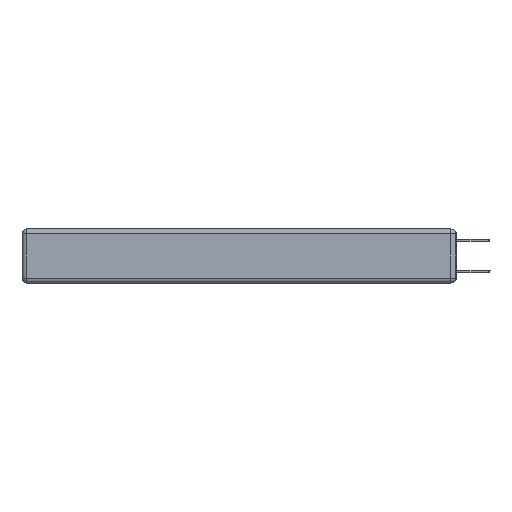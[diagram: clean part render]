
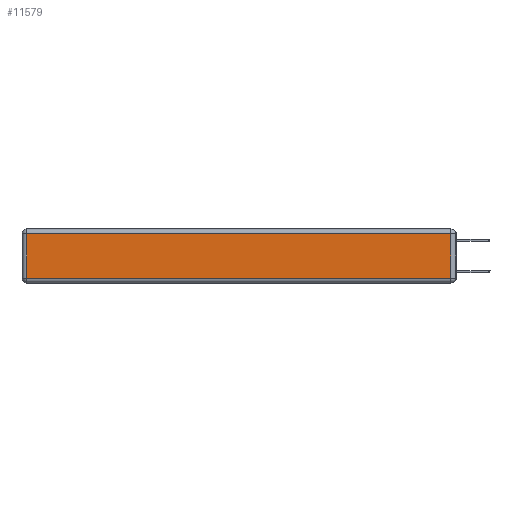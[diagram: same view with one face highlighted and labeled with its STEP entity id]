
A CAD part, left-side view. The second image highlights one B-rep face of the part: STEP entity #11579.
In plain terms, the highlighted planar face has unit normal (-1, 0, 0).
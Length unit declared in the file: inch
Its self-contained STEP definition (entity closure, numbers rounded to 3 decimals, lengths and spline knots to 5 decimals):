
#82 = CARTESIAN_POINT ( 'NONE',  ( 0., 0.03, -0.313 ) ) ;
#470 = DIRECTION ( 'NONE',  ( 0., -1., 0. ) ) ;
#1354 = ORIENTED_EDGE ( 'NONE', *, *, #13788, .T. ) ;
#1530 = AXIS2_PLACEMENT_3D ( 'NONE', #2861, #9609, #12663 ) ;
#1554 = VERTEX_POINT ( 'NONE', #12225 ) ;
#1718 = CARTESIAN_POINT ( 'NONE',  ( 0., 0., -0.313 ) ) ;
#2500 = EDGE_CURVE ( 'NONE', #9883, #1554, #4701, .T. ) ;
#2648 = DIRECTION ( 'NONE',  ( 0., 1., 0. ) ) ;
#2861 = CARTESIAN_POINT ( 'NONE',  ( 0., 0., -0.343 ) ) ;
#2983 = VECTOR ( 'NONE', #470, 39.37008 ) ;
#3297 = VECTOR ( 'NONE', #2648, 39.37008 ) ;
#3367 = CARTESIAN_POINT ( 'NONE',  ( 0., 0.03, -0.343 ) ) ;
#3409 = DIRECTION ( 'NONE',  ( 0., 0., 1. ) ) ;
#4547 = EDGE_CURVE ( 'NONE', #5683, #13073, #13888, .T. ) ;
#4701 = LINE ( 'NONE', #10184, #3297 ) ;
#5683 = VERTEX_POINT ( 'NONE', #5876 ) ;
#5876 = CARTESIAN_POINT ( 'NONE',  ( 0., 2.72, -0.313 ) ) ;
#6185 = PLANE ( 'NONE',  #1530 ) ;
#6727 = ORIENTED_EDGE ( 'NONE', *, *, #4547, .T. ) ;
#6744 = VECTOR ( 'NONE', #3409, 39.37008 ) ;
#6793 = ORIENTED_EDGE ( 'NONE', *, *, #2500, .T. ) ;
#7432 = ORIENTED_EDGE ( 'NONE', *, *, #13214, .T. ) ;
#7578 = FACE_OUTER_BOUND ( 'NONE', #11973, .T. ) ;
#8473 = VECTOR ( 'NONE', #8987, 39.37008 ) ;
#8987 = DIRECTION ( 'NONE',  ( 0., 0., -1. ) ) ;
#9609 = DIRECTION ( 'NONE',  ( -1., 0., 0. ) ) ;
#9883 = VERTEX_POINT ( 'NONE', #13950 ) ;
#10184 = CARTESIAN_POINT ( 'NONE',  ( 0., 2.75, -0.03 ) ) ;
#10312 = LINE ( 'NONE', #12172, #8473 ) ;
#11579 = ADVANCED_FACE ( 'NONE', ( #7578 ), #6185, .T. ) ;
#11973 = EDGE_LOOP ( 'NONE', ( #6727, #1354, #6793, #7432 ) ) ;
#12172 = CARTESIAN_POINT ( 'NONE',  ( 0., 2.72, -0.343 ) ) ;
#12225 = CARTESIAN_POINT ( 'NONE',  ( 0., 2.72, -0.03 ) ) ;
#12490 = LINE ( 'NONE', #3367, #6744 ) ;
#12663 = DIRECTION ( 'NONE',  ( 0., 0., 1. ) ) ;
#13073 = VERTEX_POINT ( 'NONE', #82 ) ;
#13214 = EDGE_CURVE ( 'NONE', #1554, #5683, #10312, .T. ) ;
#13788 = EDGE_CURVE ( 'NONE', #13073, #9883, #12490, .T. ) ;
#13888 = LINE ( 'NONE', #1718, #2983 ) ;
#13950 = CARTESIAN_POINT ( 'NONE',  ( 0., 0.03, -0.03 ) ) ;
